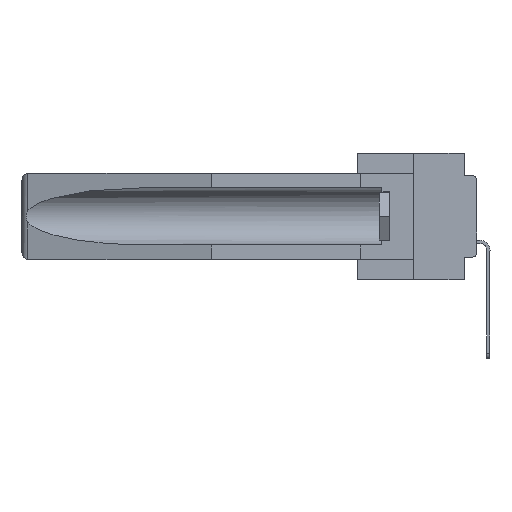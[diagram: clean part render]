
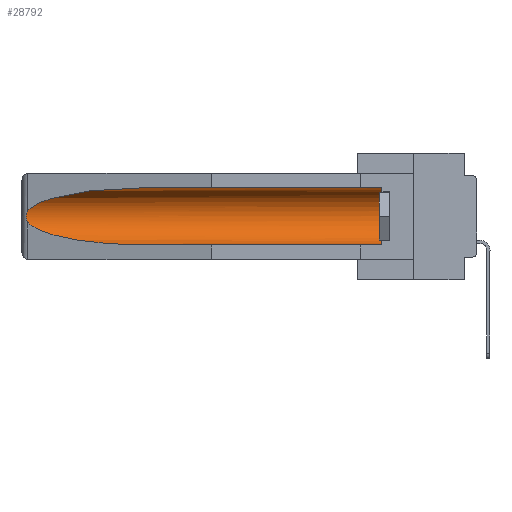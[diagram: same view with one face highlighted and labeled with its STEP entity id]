
A CAD part, left-side view. The second image highlights one B-rep face of the part: STEP entity #28792.
In plain terms, the highlighted cylindrical face has radius 2.857 mm (diameter 5.715 mm), a partial arc.
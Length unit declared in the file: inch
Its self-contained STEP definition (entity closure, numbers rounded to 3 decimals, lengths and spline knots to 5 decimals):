
#56 = CARTESIAN_POINT ( 'NONE',  ( 0.26537, 1.52718, -0.19328 ) ) ;
#3204 = VERTEX_POINT ( 'NONE', #31345 ) ;
#4316 = LINE ( 'NONE', #8955, #5469 ) ;
#4635 = ORIENTED_EDGE ( 'NONE', *, *, #8458, .T. ) ;
#5358 =( BOUNDED_CURVE ( )  B_SPLINE_CURVE ( 3, ( #16436, #21715, #24303, #24504 ),
 .UNSPECIFIED., .F., .F. ) 
 B_SPLINE_CURVE_WITH_KNOTS ( ( 4, 4 ),
 ( 4.71239, 6.08839 ),
 .UNSPECIFIED. ) 
 CURVE ( )  GEOMETRIC_REPRESENTATION_ITEM ( )  RATIONAL_B_SPLINE_CURVE ( ( 1., 0.848, 0.848, 1. ) ) 
 REPRESENTATION_ITEM ( '' )  );
#5469 = VECTOR ( 'NONE', #31552, 39.37008 ) ;
#5543 = CARTESIAN_POINT ( 'NONE',  ( 0.155, 0.126, -0.1715 ) ) ;
#6658 = ORIENTED_EDGE ( 'NONE', *, *, #14633, .T. ) ;
#7399 = CARTESIAN_POINT ( 'NONE',  ( 0.26655, 1.53094, -0.18657 ) ) ;
#7438 = ORIENTED_EDGE ( 'NONE', *, *, #11528, .F. ) ;
#7500 = CARTESIAN_POINT ( 'NONE',  ( 0.26537, 1.52718, -0.14972 ) ) ;
#8458 = EDGE_CURVE ( 'NONE', #3204, #13290, #5358, .T. ) ;
#8518 = AXIS2_PLACEMENT_3D ( 'NONE', #5543, #30933, #16020 ) ;
#8955 = CARTESIAN_POINT ( 'NONE',  ( 0.155, -0.30754, -0.284 ) ) ;
#9751 = CARTESIAN_POINT ( 'NONE',  ( 0.26537, 1.52718, -0.14972 ) ) ;
#9859 = CARTESIAN_POINT ( 'NONE',  ( 0.2673, 1.5327, -0.16383 ) ) ;
#10032 = DIRECTION ( 'NONE',  ( 0., 0., 1. ) ) ;
#10082 = CARTESIAN_POINT ( 'NONE',  ( 0.2675, 1.53308, -0.17534 ) ) ;
#11357 = VERTEX_POINT ( 'NONE', #17087 ) ;
#11528 = EDGE_CURVE ( 'NONE', #16330, #11357, #4316, .T. ) ;
#12611 = CARTESIAN_POINT ( 'NONE',  ( 0.26597, 1.5296, -0.19026 ) ) ;
#13290 = VERTEX_POINT ( 'NONE', #7500 ) ;
#13619 = CARTESIAN_POINT ( 'NONE',  ( 0.26537, 1.52718, -0.19328 ) ) ;
#14633 = EDGE_CURVE ( 'NONE', #13290, #18695, #21544, .T. ) ;
#14679 =( BOUNDED_CURVE ( )  B_SPLINE_CURVE ( 3, ( #56, #15364, #14934, #30059 ),
 .UNSPECIFIED., .F., .F. ) 
 B_SPLINE_CURVE_WITH_KNOTS ( ( 4, 4 ),
 ( 0.1948, 1.5708 ),
 .UNSPECIFIED. ) 
 CURVE ( )  GEOMETRIC_REPRESENTATION_ITEM ( )  RATIONAL_B_SPLINE_CURVE ( ( 1., 0.848, 0.848, 1. ) ) 
 REPRESENTATION_ITEM ( '' )  );
#14934 = CARTESIAN_POINT ( 'NONE',  ( 0.21114, 1.30732, -0.284 ) ) ;
#15291 = VERTEX_POINT ( 'NONE', #27922 ) ;
#15364 = CARTESIAN_POINT ( 'NONE',  ( 0.25451, 1.48313, -0.24835 ) ) ;
#16020 = DIRECTION ( 'NONE',  ( 0., 0., 1. ) ) ;
#16330 = VERTEX_POINT ( 'NONE', #19562 ) ;
#16352 = DIRECTION ( 'NONE',  ( 0., 1., 0. ) ) ;
#16436 = CARTESIAN_POINT ( 'NONE',  ( 0.155, 1.07973, -0.059 ) ) ;
#16518 = CYLINDRICAL_SURFACE ( 'NONE', #16857, 0.1125 ) ;
#16857 = AXIS2_PLACEMENT_3D ( 'NONE', #25441, #27794, #10032 ) ;
#17087 = CARTESIAN_POINT ( 'NONE',  ( 0.155, 1.07973, -0.284 ) ) ;
#17452 = CARTESIAN_POINT ( 'NONE',  ( 0.26654, 1.53092, -0.15636 ) ) ;
#18436 = EDGE_CURVE ( 'NONE', #18695, #11357, #14679, .T. ) ;
#18607 = VECTOR ( 'NONE', #16352, 39.37008 ) ;
#18695 = VERTEX_POINT ( 'NONE', #13619 ) ;
#19562 = CARTESIAN_POINT ( 'NONE',  ( 0.155, 0.126, -0.284 ) ) ;
#21544 = B_SPLINE_CURVE_WITH_KNOTS ( 'NONE', 3,
 ( #9751, #22738, #17452, #9859, #22526, #10082, #27294, #7399, #12611, #27731 ),
 .UNSPECIFIED., .F., .F.,
 ( 4, 2, 2, 2, 4 ),
 ( 0., 0.00029, 0.00058, 0.00087, 0.00117 ),
 .UNSPECIFIED. ) ;
#21715 = CARTESIAN_POINT ( 'NONE',  ( 0.21114, 1.30732, -0.059 ) ) ;
#22526 = CARTESIAN_POINT ( 'NONE',  ( 0.2675, 1.53308, -0.16763 ) ) ;
#22738 = CARTESIAN_POINT ( 'NONE',  ( 0.26597, 1.52961, -0.15275 ) ) ;
#22744 = EDGE_CURVE ( 'NONE', #16330, #15291, #25012, .T. ) ;
#23938 = ORIENTED_EDGE ( 'NONE', *, *, #27354, .T. ) ;
#24219 = CARTESIAN_POINT ( 'NONE',  ( 0.155, -0.30754, -0.059 ) ) ;
#24303 = CARTESIAN_POINT ( 'NONE',  ( 0.25451, 1.48313, -0.09465 ) ) ;
#24504 = CARTESIAN_POINT ( 'NONE',  ( 0.26537, 1.52718, -0.14972 ) ) ;
#25012 = CIRCLE ( 'NONE', #8518, 0.1125 ) ;
#25441 = CARTESIAN_POINT ( 'NONE',  ( 0.155, -0.30754, -0.1715 ) ) ;
#27294 = CARTESIAN_POINT ( 'NONE',  ( 0.2673, 1.53269, -0.17917 ) ) ;
#27354 = EDGE_CURVE ( 'NONE', #15291, #3204, #31611, .T. ) ;
#27731 = CARTESIAN_POINT ( 'NONE',  ( 0.26537, 1.52718, -0.19328 ) ) ;
#27794 = DIRECTION ( 'NONE',  ( 0., 1., 0. ) ) ;
#27922 = CARTESIAN_POINT ( 'NONE',  ( 0.155, 0.126, -0.059 ) ) ;
#28792 = ADVANCED_FACE ( 'NONE', ( #29947 ), #16518, .F. ) ;
#29586 = ORIENTED_EDGE ( 'NONE', *, *, #18436, .T. ) ;
#29760 = ORIENTED_EDGE ( 'NONE', *, *, #22744, .T. ) ;
#29947 = FACE_OUTER_BOUND ( 'NONE', #31914, .T. ) ;
#30059 = CARTESIAN_POINT ( 'NONE',  ( 0.155, 1.07973, -0.284 ) ) ;
#30933 = DIRECTION ( 'NONE',  ( 0., -1., 0. ) ) ;
#31345 = CARTESIAN_POINT ( 'NONE',  ( 0.155, 1.07973, -0.059 ) ) ;
#31552 = DIRECTION ( 'NONE',  ( 0., 1., 0. ) ) ;
#31611 = LINE ( 'NONE', #24219, #18607 ) ;
#31914 = EDGE_LOOP ( 'NONE', ( #4635, #6658, #29586, #7438, #29760, #23938 ) ) ;
